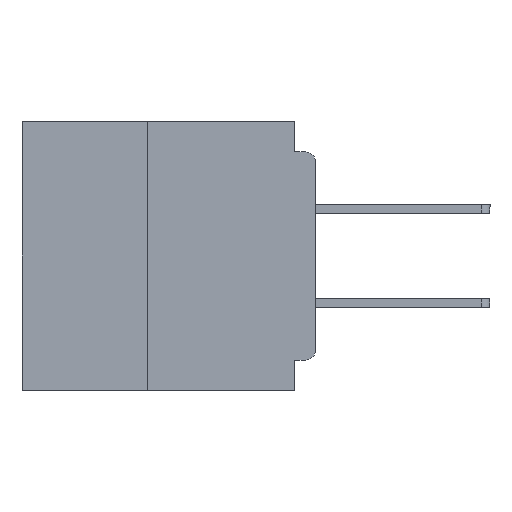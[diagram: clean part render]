
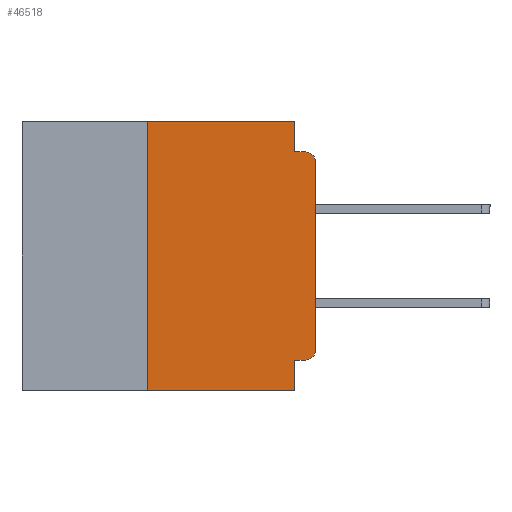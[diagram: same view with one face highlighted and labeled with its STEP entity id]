
A CAD part, left-side view. The second image highlights one B-rep face of the part: STEP entity #46518.
In plain terms, the highlighted planar face has unit normal (-1, 0, 0).
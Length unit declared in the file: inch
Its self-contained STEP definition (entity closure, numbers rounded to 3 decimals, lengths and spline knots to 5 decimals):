
#680 = VERTEX_POINT ( 'NONE', #19416 ) ;
#1365 = LINE ( 'NONE', #7033, #21391 ) ;
#1689 = LINE ( 'NONE', #36179, #41387 ) ;
#2493 = ORIENTED_EDGE ( 'NONE', *, *, #51245, .T. ) ;
#2555 = CARTESIAN_POINT ( 'NONE',  ( 0., 0.015, -0.045 ) ) ;
#2812 = CARTESIAN_POINT ( 'NONE',  ( 0., 0.031, -0.4 ) ) ;
#3126 = AXIS2_PLACEMENT_3D ( 'NONE', #31835, #8113, #35726 ) ;
#3468 = LINE ( 'NONE', #37996, #33878 ) ;
#4417 = ORIENTED_EDGE ( 'NONE', *, *, #12514, .F. ) ;
#5041 = DIRECTION ( 'NONE',  ( 1., 0., 0. ) ) ;
#5130 = VERTEX_POINT ( 'NONE', #13142 ) ;
#5674 = ORIENTED_EDGE ( 'NONE', *, *, #6591, .T. ) ;
#6591 = EDGE_CURVE ( 'NONE', #5130, #35212, #3468, .T. ) ;
#7033 = CARTESIAN_POINT ( 'NONE',  ( 0., 0.437, 0. ) ) ;
#8019 = CARTESIAN_POINT ( 'NONE',  ( 0., 0., -0.06 ) ) ;
#8059 = LINE ( 'NONE', #46697, #27965 ) ;
#8113 = DIRECTION ( 'NONE',  ( -1., 0., 0. ) ) ;
#9422 = AXIS2_PLACEMENT_3D ( 'NONE', #42522, #18927, #46459 ) ;
#10114 = ORIENTED_EDGE ( 'NONE', *, *, #43423, .F. ) ;
#10137 = EDGE_CURVE ( 'NONE', #24273, #22288, #17549, .T. ) ;
#10493 = CARTESIAN_POINT ( 'NONE',  ( 0., 0.031, -0.045 ) ) ;
#11093 = DIRECTION ( 'NONE',  ( 0., -1., 0. ) ) ;
#12514 = EDGE_CURVE ( 'NONE', #5130, #21784, #34015, .T. ) ;
#12607 = DIRECTION ( 'NONE',  ( 0., 1., 0. ) ) ;
#12641 = CARTESIAN_POINT ( 'NONE',  ( 0., 0.031, -0.355 ) ) ;
#13142 = CARTESIAN_POINT ( 'NONE',  ( 0., 0.25, -0.4 ) ) ;
#14202 = CARTESIAN_POINT ( 'NONE',  ( 0., 0., -0.34 ) ) ;
#15267 = EDGE_CURVE ( 'NONE', #33294, #46800, #46408, .T. ) ;
#16910 = ORIENTED_EDGE ( 'NONE', *, *, #36880, .F. ) ;
#16933 = PLANE ( 'NONE',  #33198 ) ;
#17549 = CIRCLE ( 'NONE', #9422, 0.015 ) ;
#18271 = VERTEX_POINT ( 'NONE', #12641 ) ;
#18512 = CARTESIAN_POINT ( 'NONE',  ( 0., 0.015, -0.355 ) ) ;
#18776 = FACE_OUTER_BOUND ( 'NONE', #23394, .T. ) ;
#18927 = DIRECTION ( 'NONE',  ( -1., 0., 0. ) ) ;
#19416 = CARTESIAN_POINT ( 'NONE',  ( 0., 0.031, 0. ) ) ;
#19569 = CARTESIAN_POINT ( 'NONE',  ( 0., 0.031, 0. ) ) ;
#21391 = VECTOR ( 'NONE', #11093, 39.37008 ) ;
#21784 = VERTEX_POINT ( 'NONE', #41821 ) ;
#22288 = VERTEX_POINT ( 'NONE', #14202 ) ;
#23394 = EDGE_LOOP ( 'NONE', ( #2493, #35406, #16910, #40360, #10114, #4417, #5674, #40996, #32996, #26309 ) ) ;
#23519 = CARTESIAN_POINT ( 'NONE',  ( 0., 0., 0. ) ) ;
#24273 = VERTEX_POINT ( 'NONE', #18512 ) ;
#25060 = VERTEX_POINT ( 'NONE', #10493 ) ;
#26309 = ORIENTED_EDGE ( 'NONE', *, *, #10137, .T. ) ;
#27965 = VECTOR ( 'NONE', #46872, 39.37008 ) ;
#28888 = CARTESIAN_POINT ( 'NONE',  ( 0., 0.437, 0. ) ) ;
#29769 = DIRECTION ( 'NONE',  ( 0., 0., 1. ) ) ;
#31607 = VECTOR ( 'NONE', #29769, 39.37008 ) ;
#31835 = CARTESIAN_POINT ( 'NONE',  ( 0., 0.015, -0.06 ) ) ;
#32653 = LINE ( 'NONE', #2812, #41895 ) ;
#32797 = DIRECTION ( 'NONE',  ( 0., 0., -1. ) ) ;
#32996 = ORIENTED_EDGE ( 'NONE', *, *, #48637, .F. ) ;
#33198 = AXIS2_PLACEMENT_3D ( 'NONE', #28888, #5041, #32797 ) ;
#33294 = VERTEX_POINT ( 'NONE', #8019 ) ;
#33878 = VECTOR ( 'NONE', #34202, 39.37008 ) ;
#34015 = LINE ( 'NONE', #37620, #31607 ) ;
#34202 = DIRECTION ( 'NONE',  ( 0., -1., 0. ) ) ;
#34555 = DIRECTION ( 'NONE',  ( 0., 0., -1. ) ) ;
#35212 = VERTEX_POINT ( 'NONE', #35807 ) ;
#35406 = ORIENTED_EDGE ( 'NONE', *, *, #15267, .T. ) ;
#35726 = DIRECTION ( 'NONE',  ( 0., 0., -1. ) ) ;
#35807 = CARTESIAN_POINT ( 'NONE',  ( 0., 0.031, -0.4 ) ) ;
#36179 = CARTESIAN_POINT ( 'NONE',  ( 0., 0., -0.355 ) ) ;
#36880 = EDGE_CURVE ( 'NONE', #25060, #46800, #8059, .T. ) ;
#37038 = LINE ( 'NONE', #23519, #38317 ) ;
#37620 = CARTESIAN_POINT ( 'NONE',  ( 0., 0.25, -0.4 ) ) ;
#37996 = CARTESIAN_POINT ( 'NONE',  ( 0., 0.437, -0.4 ) ) ;
#38080 = LINE ( 'NONE', #19569, #48543 ) ;
#38317 = VECTOR ( 'NONE', #50910, 39.37008 ) ;
#40360 = ORIENTED_EDGE ( 'NONE', *, *, #50640, .F. ) ;
#40996 = ORIENTED_EDGE ( 'NONE', *, *, #49676, .F. ) ;
#41387 = VECTOR ( 'NONE', #12607, 39.37008 ) ;
#41821 = CARTESIAN_POINT ( 'NONE',  ( 0., 0.25, 0. ) ) ;
#41895 = VECTOR ( 'NONE', #34555, 39.37008 ) ;
#42522 = CARTESIAN_POINT ( 'NONE',  ( 0., 0.015, -0.34 ) ) ;
#43423 = EDGE_CURVE ( 'NONE', #21784, #680, #1365, .T. ) ;
#46408 = CIRCLE ( 'NONE', #3126, 0.015 ) ;
#46459 = DIRECTION ( 'NONE',  ( 0., 0., -1. ) ) ;
#46518 = ADVANCED_FACE ( 'NONE', ( #18776 ), #16933, .F. ) ;
#46697 = CARTESIAN_POINT ( 'NONE',  ( 0., 0., -0.045 ) ) ;
#46800 = VERTEX_POINT ( 'NONE', #2555 ) ;
#46872 = DIRECTION ( 'NONE',  ( 0., -1., 0. ) ) ;
#48543 = VECTOR ( 'NONE', #50970, 39.37008 ) ;
#48637 = EDGE_CURVE ( 'NONE', #24273, #18271, #1689, .T. ) ;
#49676 = EDGE_CURVE ( 'NONE', #18271, #35212, #32653, .T. ) ;
#50640 = EDGE_CURVE ( 'NONE', #680, #25060, #38080, .T. ) ;
#50910 = DIRECTION ( 'NONE',  ( 0., 0., 1. ) ) ;
#50970 = DIRECTION ( 'NONE',  ( 0., 0., -1. ) ) ;
#51245 = EDGE_CURVE ( 'NONE', #22288, #33294, #37038, .T. ) ;
